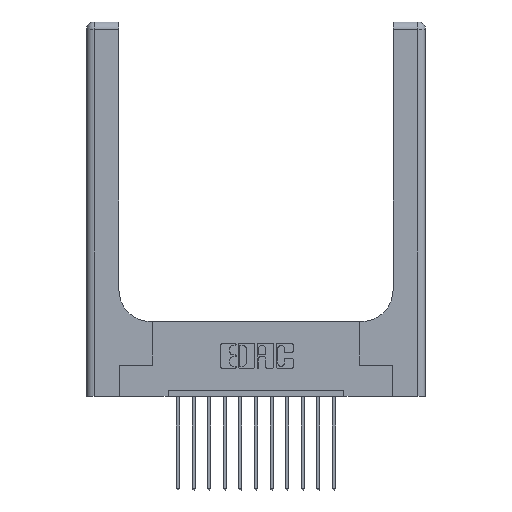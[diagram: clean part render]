
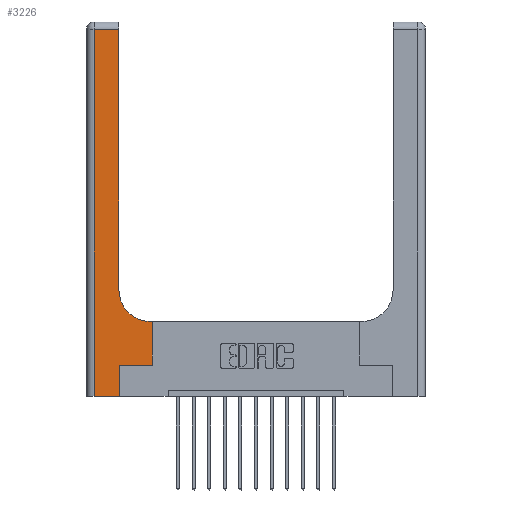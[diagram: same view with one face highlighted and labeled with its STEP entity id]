
A CAD part, top view. The second image highlights one B-rep face of the part: STEP entity #3226.
In plain terms, the highlighted planar face has unit normal (0, 0, 1).
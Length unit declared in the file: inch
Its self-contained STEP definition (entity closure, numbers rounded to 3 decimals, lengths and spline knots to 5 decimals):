
#477 = DIRECTION ( 'NONE',  ( 1., 0., 0. ) ) ;
#1564 = FACE_OUTER_BOUND ( 'NONE', #13938, .T. ) ;
#1698 = VERTEX_POINT ( 'NONE', #15223 ) ;
#1852 = EDGE_CURVE ( 'NONE', #1698, #14673, #4945, .T. ) ;
#2351 = CARTESIAN_POINT ( 'NONE',  ( 0.265, 0., 0.37 ) ) ;
#2368 = EDGE_CURVE ( 'NONE', #12087, #5290, #12787, .T. ) ;
#2798 = ORIENTED_EDGE ( 'NONE', *, *, #4500, .T. ) ;
#2849 = AXIS2_PLACEMENT_3D ( 'NONE', #3510, #14700, #4803 ) ;
#3121 = DIRECTION ( 'NONE',  ( -1., 0., 0. ) ) ;
#3179 = LINE ( 'NONE', #14855, #7695 ) ;
#3226 = ADVANCED_FACE ( 'NONE', ( #1564 ), #3249, .F. ) ;
#3249 = PLANE ( 'NONE',  #2849 ) ;
#3334 = LINE ( 'NONE', #8240, #14688 ) ;
#3490 = CARTESIAN_POINT ( 'NONE',  ( 0.26, 0.85, 0.37 ) ) ;
#3510 = CARTESIAN_POINT ( 'NONE',  ( 0., 3., 0.37 ) ) ;
#3699 = LINE ( 'NONE', #6729, #10175 ) ;
#3723 = CARTESIAN_POINT ( 'NONE',  ( 0.265, 0.25, 0.37 ) ) ;
#4148 = CARTESIAN_POINT ( 'NONE',  ( 0.06, 3., 0.37 ) ) ;
#4432 = VERTEX_POINT ( 'NONE', #15938 ) ;
#4479 = EDGE_CURVE ( 'NONE', #8518, #4432, #13692, .T. ) ;
#4500 = EDGE_CURVE ( 'NONE', #4432, #4782, #5058, .T. ) ;
#4782 = VERTEX_POINT ( 'NONE', #11075 ) ;
#4803 = DIRECTION ( 'NONE',  ( -1., 0., 0. ) ) ;
#4860 = VECTOR ( 'NONE', #8455, 39.37008 ) ;
#4863 = DIRECTION ( 'NONE',  ( 0., 1., 0. ) ) ;
#4945 = CIRCLE ( 'NONE', #10638, 0.25 ) ;
#5058 = LINE ( 'NONE', #14802, #14631 ) ;
#5104 = ORIENTED_EDGE ( 'NONE', *, *, #4479, .T. ) ;
#5135 = DIRECTION ( 'NONE',  ( 0., 1., 0. ) ) ;
#5137 = CARTESIAN_POINT ( 'NONE',  ( 0.06, 2.94, 0.37 ) ) ;
#5290 = VERTEX_POINT ( 'NONE', #2351 ) ;
#5429 = VECTOR ( 'NONE', #5135, 39.37008 ) ;
#5708 = ORIENTED_EDGE ( 'NONE', *, *, #11196, .T. ) ;
#5833 = ORIENTED_EDGE ( 'NONE', *, *, #13888, .T. ) ;
#5858 = CARTESIAN_POINT ( 'NONE',  ( 0.265, 0.25, 0.37 ) ) ;
#6445 = CARTESIAN_POINT ( 'NONE',  ( 0.265, 0., 0.37 ) ) ;
#6458 = ORIENTED_EDGE ( 'NONE', *, *, #2368, .T. ) ;
#6729 = CARTESIAN_POINT ( 'NONE',  ( 0., 2.94, 0.37 ) ) ;
#6926 = CARTESIAN_POINT ( 'NONE',  ( 0.51, 0.85, 0.37 ) ) ;
#7006 = DIRECTION ( 'NONE',  ( 1., 0., 0. ) ) ;
#7553 = ORIENTED_EDGE ( 'NONE', *, *, #1852, .T. ) ;
#7695 = VECTOR ( 'NONE', #11370, 39.37008 ) ;
#7822 = VECTOR ( 'NONE', #7884, 39.37008 ) ;
#7884 = DIRECTION ( 'NONE',  ( 0., -1., 0. ) ) ;
#8240 = CARTESIAN_POINT ( 'NONE',  ( 0.26, 0.6, 0.37 ) ) ;
#8455 = DIRECTION ( 'NONE',  ( 1., 0., 0. ) ) ;
#8518 = VERTEX_POINT ( 'NONE', #3723 ) ;
#9098 = EDGE_CURVE ( 'NONE', #14673, #11366, #3179, .T. ) ;
#10175 = VECTOR ( 'NONE', #14414, 39.37008 ) ;
#10638 = AXIS2_PLACEMENT_3D ( 'NONE', #6926, #13197, #477 ) ;
#10688 = ORIENTED_EDGE ( 'NONE', *, *, #9098, .T. ) ;
#11075 = CARTESIAN_POINT ( 'NONE',  ( 0.528, 0.6, 0.37 ) ) ;
#11196 = EDGE_CURVE ( 'NONE', #11366, #13304, #3699, .T. ) ;
#11366 = VERTEX_POINT ( 'NONE', #13209 ) ;
#11370 = DIRECTION ( 'NONE',  ( 0., 1., 0. ) ) ;
#11910 = CARTESIAN_POINT ( 'NONE',  ( 0., 0., 0.37 ) ) ;
#12024 = EDGE_CURVE ( 'NONE', #5290, #8518, #15575, .T. ) ;
#12087 = VERTEX_POINT ( 'NONE', #14087 ) ;
#12787 = LINE ( 'NONE', #11910, #15103 ) ;
#12907 = ORIENTED_EDGE ( 'NONE', *, *, #15332, .T. ) ;
#13197 = DIRECTION ( 'NONE',  ( 0., 0., -1. ) ) ;
#13209 = CARTESIAN_POINT ( 'NONE',  ( 0.26, 2.94, 0.37 ) ) ;
#13304 = VERTEX_POINT ( 'NONE', #5137 ) ;
#13664 = LINE ( 'NONE', #4148, #7822 ) ;
#13692 = LINE ( 'NONE', #5858, #4860 ) ;
#13888 = EDGE_CURVE ( 'NONE', #4782, #1698, #3334, .T. ) ;
#13938 = EDGE_LOOP ( 'NONE', ( #10688, #5708, #12907, #6458, #15384, #5104, #2798, #5833, #7553 ) ) ;
#14087 = CARTESIAN_POINT ( 'NONE',  ( 0.06, 0., 0.37 ) ) ;
#14414 = DIRECTION ( 'NONE',  ( -1., 0., 0. ) ) ;
#14631 = VECTOR ( 'NONE', #4863, 39.37008 ) ;
#14673 = VERTEX_POINT ( 'NONE', #3490 ) ;
#14688 = VECTOR ( 'NONE', #3121, 39.37008 ) ;
#14700 = DIRECTION ( 'NONE',  ( 0., 0., -1. ) ) ;
#14802 = CARTESIAN_POINT ( 'NONE',  ( 0.528, 0.25, 0.37 ) ) ;
#14855 = CARTESIAN_POINT ( 'NONE',  ( 0.26, 3., 0.37 ) ) ;
#15103 = VECTOR ( 'NONE', #7006, 39.37008 ) ;
#15223 = CARTESIAN_POINT ( 'NONE',  ( 0.51, 0.6, 0.37 ) ) ;
#15332 = EDGE_CURVE ( 'NONE', #13304, #12087, #13664, .T. ) ;
#15384 = ORIENTED_EDGE ( 'NONE', *, *, #12024, .T. ) ;
#15575 = LINE ( 'NONE', #6445, #5429 ) ;
#15938 = CARTESIAN_POINT ( 'NONE',  ( 0.528, 0.25, 0.37 ) ) ;
